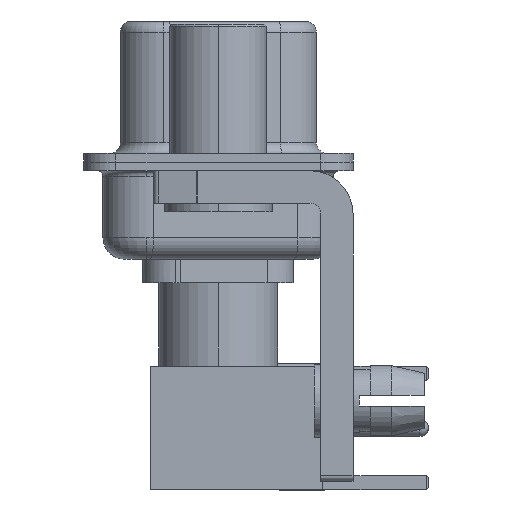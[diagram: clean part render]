
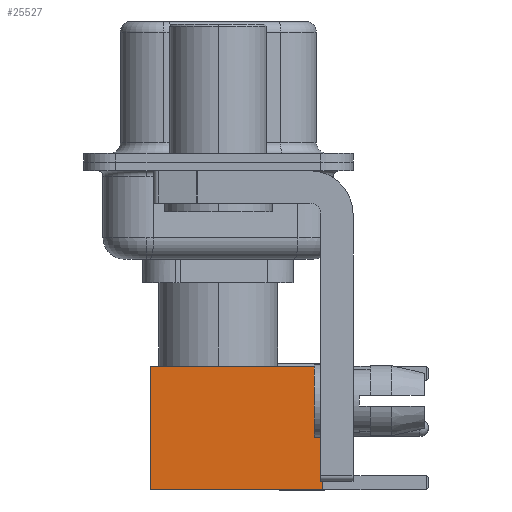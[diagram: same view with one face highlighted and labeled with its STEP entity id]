
A CAD part, left-side view. The second image highlights one B-rep face of the part: STEP entity #25527.
In plain terms, the highlighted face is planar.
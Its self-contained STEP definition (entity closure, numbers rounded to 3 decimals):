
#3840 = ORIENTED_EDGE ( 'NONE', *, *, #22116, .T. ) ;
#4934 = CARTESIAN_POINT ( 'NONE',  ( -2.875, 2.875, 8. ) ) ;
#5213 = CARTESIAN_POINT ( 'NONE',  ( 0., 2.875, 0. ) ) ;
#8208 = ORIENTED_EDGE ( 'NONE', *, *, #8615, .F. ) ;
#8615 = EDGE_CURVE ( 'NONE', #14029, #31300, #26985, .T. ) ;
#8762 = ORIENTED_EDGE ( 'NONE', *, *, #28006, .T. ) ;
#10329 = VERTEX_POINT ( 'NONE', #19768 ) ;
#10454 = DIRECTION ( 'NONE',  ( 0., 1., 0. ) ) ;
#10553 = CARTESIAN_POINT ( 'NONE',  ( 0., 2.875, 8. ) ) ;
#11431 = DIRECTION ( 'NONE',  ( 0., 0., -1. ) ) ;
#13338 = CARTESIAN_POINT ( 'NONE',  ( -2.875, 2.875, 0. ) ) ;
#13797 = CARTESIAN_POINT ( 'NONE',  ( -2.875, 2.875, 0. ) ) ;
#14029 = VERTEX_POINT ( 'NONE', #20079 ) ;
#14259 = LINE ( 'NONE', #13797, #23895 ) ;
#15050 = DIRECTION ( 'NONE',  ( 0., 0., 1. ) ) ;
#16750 = CARTESIAN_POINT ( 'NONE',  ( 2.875, 2.875, 0. ) ) ;
#17533 = EDGE_CURVE ( 'NONE', #31300, #23795, #14259, .T. ) ;
#17618 = AXIS2_PLACEMENT_3D ( 'NONE', #29264, #10454, #15050 ) ;
#17635 = LINE ( 'NONE', #5213, #25641 ) ;
#19768 = CARTESIAN_POINT ( 'NONE',  ( 2.875, 2.875, 0. ) ) ;
#20079 = CARTESIAN_POINT ( 'NONE',  ( 2.875, 2.875, 8. ) ) ;
#20177 = FACE_OUTER_BOUND ( 'NONE', #28241, .T. ) ;
#20280 = DIRECTION ( 'NONE',  ( -1., 0., 0. ) ) ;
#22116 = EDGE_CURVE ( 'NONE', #10329, #23795, #17635, .T. ) ;
#22588 = DIRECTION ( 'NONE',  ( -1., 0., 0. ) ) ;
#23627 = DIRECTION ( 'NONE',  ( 0., 0., -1. ) ) ;
#23795 = VERTEX_POINT ( 'NONE', #13338 ) ;
#23895 = VECTOR ( 'NONE', #11431, 1000. ) ;
#25527 = ADVANCED_FACE ( 'NONE', ( #20177 ), #27339, .T. ) ;
#25641 = VECTOR ( 'NONE', #22588, 1000. ) ;
#26162 = LINE ( 'NONE', #16750, #28421 ) ;
#26761 = VECTOR ( 'NONE', #20280, 1000. ) ;
#26985 = LINE ( 'NONE', #10553, #26761 ) ;
#27339 = PLANE ( 'NONE',  #17618 ) ;
#28006 = EDGE_CURVE ( 'NONE', #14029, #10329, #26162, .T. ) ;
#28241 = EDGE_LOOP ( 'NONE', ( #8762, #3840, #29385, #8208 ) ) ;
#28421 = VECTOR ( 'NONE', #23627, 1000. ) ;
#29264 = CARTESIAN_POINT ( 'NONE',  ( 2.875, 2.875, 0. ) ) ;
#29385 = ORIENTED_EDGE ( 'NONE', *, *, #17533, .F. ) ;
#31300 = VERTEX_POINT ( 'NONE', #4934 ) ;
